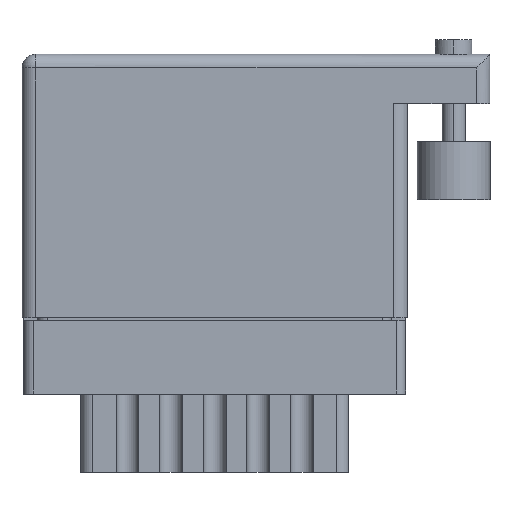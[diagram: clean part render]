
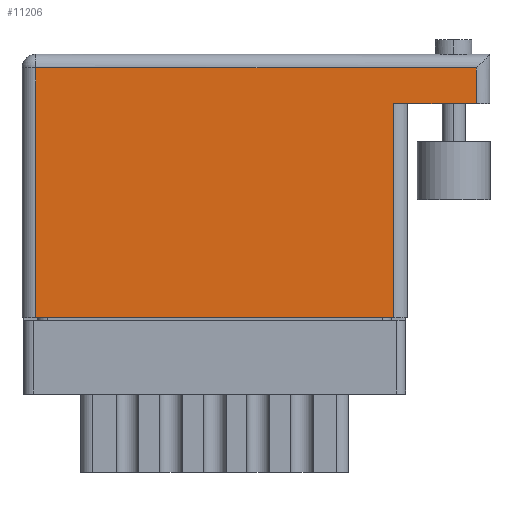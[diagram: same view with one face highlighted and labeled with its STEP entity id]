
A CAD part, front view. The second image highlights one B-rep face of the part: STEP entity #11206.
In plain terms, the highlighted face is planar.
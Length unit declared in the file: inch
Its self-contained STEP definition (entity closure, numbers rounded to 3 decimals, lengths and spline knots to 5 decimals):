
#203 = DIRECTION ( 'NONE',  ( 1., 0., 0. ) ) ;
#702 = CARTESIAN_POINT ( 'NONE',  ( 1.562, 0.736, 0. ) ) ;
#865 = VERTEX_POINT ( 'NONE', #2521 ) ;
#1478 = DIRECTION ( 'NONE',  ( 0., 1., 0. ) ) ;
#1519 = EDGE_CURVE ( 'NONE', #8493, #865, #2621, .T. ) ;
#1574 = CARTESIAN_POINT ( 'NONE',  ( 1.562, 0.859, 0. ) ) ;
#1714 = CARTESIAN_POINT ( 'NONE',  ( 0.047, 0.859, 0. ) ) ;
#1938 = LINE ( 'NONE', #9997, #24871 ) ;
#2344 = LINE ( 'NONE', #9750, #15772 ) ;
#2521 = CARTESIAN_POINT ( 'NONE',  ( 1.278, 0.736, 0. ) ) ;
#2552 = CARTESIAN_POINT ( 'NONE',  ( 1.609, 0.736, 0. ) ) ;
#2621 = LINE ( 'NONE', #2552, #10813 ) ;
#2716 = ORIENTED_EDGE ( 'NONE', *, *, #1519, .F. ) ;
#3897 = FACE_OUTER_BOUND ( 'NONE', #19486, .T. ) ;
#5180 = ORIENTED_EDGE ( 'NONE', *, *, #21129, .T. ) ;
#5452 = PLANE ( 'NONE',  #6505 ) ;
#5456 = LINE ( 'NONE', #24748, #21167 ) ;
#5967 = ORIENTED_EDGE ( 'NONE', *, *, #17657, .T. ) ;
#6277 = VERTEX_POINT ( 'NONE', #27143 ) ;
#6393 = CARTESIAN_POINT ( 'NONE',  ( 0., 0., 0. ) ) ;
#6505 = AXIS2_PLACEMENT_3D ( 'NONE', #20073, #15507, #9311 ) ;
#6766 = EDGE_CURVE ( 'NONE', #8493, #7734, #1938, .T. ) ;
#6885 = VERTEX_POINT ( 'NONE', #27020 ) ;
#7703 = EDGE_CURVE ( 'NONE', #7734, #12146, #18247, .T. ) ;
#7734 = VERTEX_POINT ( 'NONE', #1574 ) ;
#8493 = VERTEX_POINT ( 'NONE', #702 ) ;
#9311 = DIRECTION ( 'NONE',  ( -1., 0., 0. ) ) ;
#9750 = CARTESIAN_POINT ( 'NONE',  ( 1.278, 0.736, 0. ) ) ;
#9997 = CARTESIAN_POINT ( 'NONE',  ( 1.562, 0.906, 0. ) ) ;
#10813 = VECTOR ( 'NONE', #19004, 39.37008 ) ;
#11206 = ADVANCED_FACE ( 'NONE', ( #3897 ), #5452, .F. ) ;
#12146 = VERTEX_POINT ( 'NONE', #1714 ) ;
#12256 = ORIENTED_EDGE ( 'NONE', *, *, #25871, .T. ) ;
#14019 = DIRECTION ( 'NONE',  ( -1., 0., 0. ) ) ;
#14373 = CARTESIAN_POINT ( 'NONE',  ( 0., 0.859, 0. ) ) ;
#15324 = VECTOR ( 'NONE', #14019, 39.37008 ) ;
#15507 = DIRECTION ( 'NONE',  ( 0., 0., -1. ) ) ;
#15772 = VECTOR ( 'NONE', #18129, 39.37008 ) ;
#17089 = ORIENTED_EDGE ( 'NONE', *, *, #6766, .T. ) ;
#17657 = EDGE_CURVE ( 'NONE', #12146, #6885, #5456, .T. ) ;
#18129 = DIRECTION ( 'NONE',  ( 0., 1., 0. ) ) ;
#18247 = LINE ( 'NONE', #14373, #15324 ) ;
#19004 = DIRECTION ( 'NONE',  ( -1., 0., 0. ) ) ;
#19486 = EDGE_LOOP ( 'NONE', ( #12256, #5180, #2716, #17089, #22394, #5967 ) ) ;
#20073 = CARTESIAN_POINT ( 'NONE',  ( 0., 0.906, 0. ) ) ;
#20975 = VECTOR ( 'NONE', #203, 39.37008 ) ;
#21129 = EDGE_CURVE ( 'NONE', #6277, #865, #2344, .T. ) ;
#21167 = VECTOR ( 'NONE', #26870, 39.37008 ) ;
#22394 = ORIENTED_EDGE ( 'NONE', *, *, #7703, .T. ) ;
#24748 = CARTESIAN_POINT ( 'NONE',  ( 0.047, 0., 0. ) ) ;
#24871 = VECTOR ( 'NONE', #1478, 39.37008 ) ;
#25871 = EDGE_CURVE ( 'NONE', #6885, #6277, #26269, .T. ) ;
#26269 = LINE ( 'NONE', #6393, #20975 ) ;
#26870 = DIRECTION ( 'NONE',  ( 0., -1., 0. ) ) ;
#27020 = CARTESIAN_POINT ( 'NONE',  ( 0.047, 0., 0. ) ) ;
#27143 = CARTESIAN_POINT ( 'NONE',  ( 1.278, 0., 0. ) ) ;
